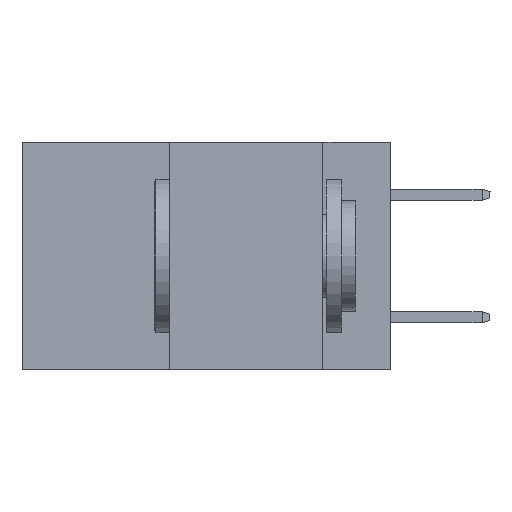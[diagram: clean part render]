
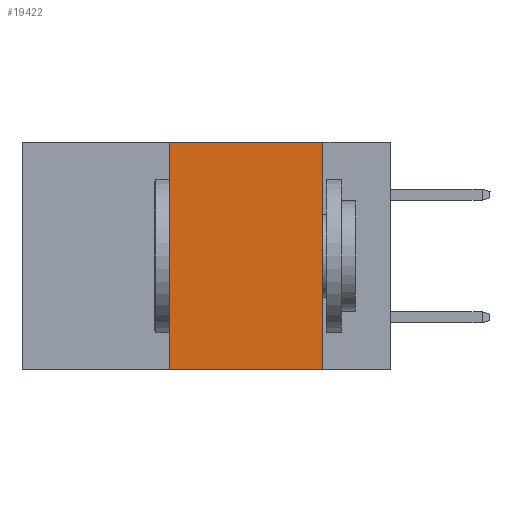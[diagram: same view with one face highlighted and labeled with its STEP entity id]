
A CAD part, left-side view. The second image highlights one B-rep face of the part: STEP entity #19422.
In plain terms, the highlighted planar face has unit normal (-1, 0, 0).
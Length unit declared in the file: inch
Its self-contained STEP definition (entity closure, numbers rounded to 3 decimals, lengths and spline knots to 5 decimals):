
#345 = DIRECTION ( 'NONE',  ( 0., 0., -1. ) ) ;
#448 = EDGE_CURVE ( 'NONE', #2863, #25835, #28439, .T. ) ;
#2863 = VERTEX_POINT ( 'NONE', #20352 ) ;
#4176 = CARTESIAN_POINT ( 'NONE',  ( 0., 0.6, -0.37 ) ) ;
#4210 = VECTOR ( 'NONE', #8661, 39.37008 ) ;
#6388 = CARTESIAN_POINT ( 'NONE',  ( 0., 0.36, 0. ) ) ;
#6528 = LINE ( 'NONE', #36533, #13765 ) ;
#7503 = VECTOR ( 'NONE', #25486, 39.37008 ) ;
#7576 = VERTEX_POINT ( 'NONE', #30303 ) ;
#7809 = DIRECTION ( 'NONE',  ( 0., 0., -1. ) ) ;
#8661 = DIRECTION ( 'NONE',  ( 0., 0., 1. ) ) ;
#12001 = VERTEX_POINT ( 'NONE', #24795 ) ;
#13765 = VECTOR ( 'NONE', #345, 39.37008 ) ;
#14314 = ORIENTED_EDGE ( 'NONE', *, *, #26516, .T. ) ;
#14770 = LINE ( 'NONE', #4176, #7503 ) ;
#15200 = FACE_OUTER_BOUND ( 'NONE', #29006, .T. ) ;
#16006 = AXIS2_PLACEMENT_3D ( 'NONE', #31859, #26048, #7809 ) ;
#16993 = PLANE ( 'NONE',  #16006 ) ;
#17840 = DIRECTION ( 'NONE',  ( 0., -1., 0. ) ) ;
#19422 = ADVANCED_FACE ( 'NONE', ( #15200 ), #16993, .F. ) ;
#20272 = EDGE_CURVE ( 'NONE', #25835, #12001, #37900, .T. ) ;
#20352 = CARTESIAN_POINT ( 'NONE',  ( 0., 0.36, -0.37 ) ) ;
#24693 = ORIENTED_EDGE ( 'NONE', *, *, #27020, .F. ) ;
#24795 = CARTESIAN_POINT ( 'NONE',  ( 0., 0.11, 0. ) ) ;
#25486 = DIRECTION ( 'NONE',  ( 0., -1., 0. ) ) ;
#25835 = VERTEX_POINT ( 'NONE', #31486 ) ;
#26048 = DIRECTION ( 'NONE',  ( 1., 0., 0. ) ) ;
#26516 = EDGE_CURVE ( 'NONE', #2863, #7576, #14770, .T. ) ;
#27020 = EDGE_CURVE ( 'NONE', #12001, #7576, #6528, .T. ) ;
#28429 = ORIENTED_EDGE ( 'NONE', *, *, #448, .F. ) ;
#28439 = LINE ( 'NONE', #6388, #4210 ) ;
#29006 = EDGE_LOOP ( 'NONE', ( #24693, #34421, #28429, #14314 ) ) ;
#30096 = VECTOR ( 'NONE', #17840, 39.37008 ) ;
#30303 = CARTESIAN_POINT ( 'NONE',  ( 0., 0.11, -0.37 ) ) ;
#31486 = CARTESIAN_POINT ( 'NONE',  ( 0., 0.36, 0. ) ) ;
#31859 = CARTESIAN_POINT ( 'NONE',  ( 0., 0.6, 0. ) ) ;
#32705 = CARTESIAN_POINT ( 'NONE',  ( 0., 0.6, 0. ) ) ;
#34421 = ORIENTED_EDGE ( 'NONE', *, *, #20272, .F. ) ;
#36533 = CARTESIAN_POINT ( 'NONE',  ( 0., 0.11, 0. ) ) ;
#37900 = LINE ( 'NONE', #32705, #30096 ) ;
